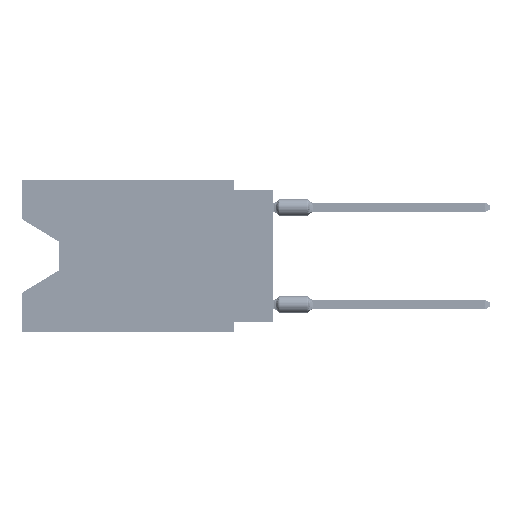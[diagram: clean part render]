
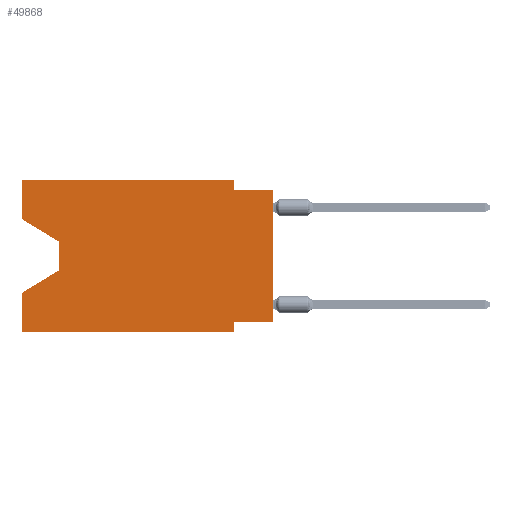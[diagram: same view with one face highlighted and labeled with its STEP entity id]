
A CAD part, left-side view. The second image highlights one B-rep face of the part: STEP entity #49868.
In plain terms, the highlighted planar face has unit normal (-1, 0, 0).
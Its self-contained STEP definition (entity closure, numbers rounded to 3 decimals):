
#768 = EDGE_CURVE ( 'NONE', #69960, #24962, #81163, .T. ) ;
#1006 = EDGE_CURVE ( 'NONE', #70549, #54076, #15546, .T. ) ;
#4411 = ORIENTED_EDGE ( 'NONE', *, *, #64118, .T. ) ;
#5309 = VECTOR ( 'NONE', #42907, 1000. ) ;
#5579 = CARTESIAN_POINT ( 'NONE',  ( 0., 2.54, -0.635 ) ) ;
#6968 = ORIENTED_EDGE ( 'NONE', *, *, #57797, .T. ) ;
#8284 = DIRECTION ( 'NONE',  ( 1., 0., 0. ) ) ;
#9071 = DIRECTION ( 'NONE',  ( 0., 0., -1. ) ) ;
#11226 = CARTESIAN_POINT ( 'NONE',  ( 0., 0., -0.635 ) ) ;
#12675 = VERTEX_POINT ( 'NONE', #26516 ) ;
#13913 = ORIENTED_EDGE ( 'NONE', *, *, #57870, .T. ) ;
#14040 = EDGE_CURVE ( 'NONE', #12675, #62823, #24757, .T. ) ;
#14303 = DIRECTION ( 'NONE',  ( 0., 1., 0. ) ) ;
#14999 = PLANE ( 'NONE',  #27653 ) ;
#15546 = LINE ( 'NONE', #59275, #26332 ) ;
#15620 = VECTOR ( 'NONE', #56709, 1000. ) ;
#15772 = VERTEX_POINT ( 'NONE', #11226 ) ;
#17292 = CARTESIAN_POINT ( 'NONE',  ( 0., 16.383, -9.906 ) ) ;
#17802 = CARTESIAN_POINT ( 'NONE',  ( 0., 13.97, -5.893 ) ) ;
#19247 = CARTESIAN_POINT ( 'NONE',  ( 0., 2.54, -9.906 ) ) ;
#19564 = LINE ( 'NONE', #26283, #22135 ) ;
#22135 = VECTOR ( 'NONE', #33429, 1000. ) ;
#23839 = DIRECTION ( 'NONE',  ( 0., 0., 1. ) ) ;
#24064 = VERTEX_POINT ( 'NONE', #17802 ) ;
#24757 = LINE ( 'NONE', #44124, #15620 ) ;
#24962 = VERTEX_POINT ( 'NONE', #19247 ) ;
#25573 = EDGE_CURVE ( 'NONE', #70549, #15772, #19564, .T. ) ;
#25638 = CARTESIAN_POINT ( 'NONE',  ( 0., 16.383, 0. ) ) ;
#25641 = LINE ( 'NONE', #70570, #53686 ) ;
#26283 = CARTESIAN_POINT ( 'NONE',  ( 0., 0., 0. ) ) ;
#26332 = VECTOR ( 'NONE', #14303, 1000. ) ;
#26516 = CARTESIAN_POINT ( 'NONE',  ( 0., 2.54, 0. ) ) ;
#27653 = AXIS2_PLACEMENT_3D ( 'NONE', #40669, #8284, #28854 ) ;
#28854 = DIRECTION ( 'NONE',  ( 0., 0., -1. ) ) ;
#29855 = LINE ( 'NONE', #55498, #5309 ) ;
#32883 = DIRECTION ( 'NONE',  ( 0., 0.855, -0.519 ) ) ;
#33429 = DIRECTION ( 'NONE',  ( 0., 0., 1. ) ) ;
#33769 = EDGE_CURVE ( 'NONE', #51291, #51063, #41152, .T. ) ;
#34732 = EDGE_CURVE ( 'NONE', #69960, #39085, #69340, .T. ) ;
#35984 = VERTEX_POINT ( 'NONE', #67940 ) ;
#38389 = ORIENTED_EDGE ( 'NONE', *, *, #25573, .T. ) ;
#39085 = VERTEX_POINT ( 'NONE', #78237 ) ;
#39200 = CARTESIAN_POINT ( 'NONE',  ( 0., 13.97, -5.893 ) ) ;
#40669 = CARTESIAN_POINT ( 'NONE',  ( 0., 16.383, 0. ) ) ;
#41152 = LINE ( 'NONE', #81413, #45690 ) ;
#42014 = VECTOR ( 'NONE', #80746, 1000. ) ;
#42800 = ORIENTED_EDGE ( 'NONE', *, *, #768, .T. ) ;
#42907 = DIRECTION ( 'NONE',  ( 0., -0.855, -0.519 ) ) ;
#43771 = VECTOR ( 'NONE', #61012, 1000. ) ;
#44076 = ORIENTED_EDGE ( 'NONE', *, *, #33769, .F. ) ;
#44124 = CARTESIAN_POINT ( 'NONE',  ( 0., 2.54, 0. ) ) ;
#44473 = ORIENTED_EDGE ( 'NONE', *, *, #80809, .F. ) ;
#44605 = EDGE_CURVE ( 'NONE', #62823, #15772, #48021, .T. ) ;
#45084 = ORIENTED_EDGE ( 'NONE', *, *, #34732, .F. ) ;
#45395 = DIRECTION ( 'NONE',  ( 0., 0., -1. ) ) ;
#45690 = VECTOR ( 'NONE', #23839, 1000. ) ;
#47388 = FACE_OUTER_BOUND ( 'NONE', #77397, .T. ) ;
#47866 = ORIENTED_EDGE ( 'NONE', *, *, #44605, .F. ) ;
#48021 = LINE ( 'NONE', #55122, #42014 ) ;
#48930 = CARTESIAN_POINT ( 'NONE',  ( 0., 16.383, 0. ) ) ;
#49868 = ADVANCED_FACE ( 'NONE', ( #47388 ), #14999, .F. ) ;
#51063 = VERTEX_POINT ( 'NONE', #65012 ) ;
#51291 = VERTEX_POINT ( 'NONE', #75471 ) ;
#53686 = VECTOR ( 'NONE', #45395, 1000. ) ;
#54076 = VERTEX_POINT ( 'NONE', #82957 ) ;
#55122 = CARTESIAN_POINT ( 'NONE',  ( 0., 0., -0.635 ) ) ;
#55498 = CARTESIAN_POINT ( 'NONE',  ( 0., 16.383, -2.546 ) ) ;
#56709 = DIRECTION ( 'NONE',  ( 0., 0., -1. ) ) ;
#57797 = EDGE_CURVE ( 'NONE', #51291, #35984, #29855, .T. ) ;
#57870 = EDGE_CURVE ( 'NONE', #35984, #24064, #25641, .T. ) ;
#58385 = DIRECTION ( 'NONE',  ( 0., 0., 1. ) ) ;
#59275 = CARTESIAN_POINT ( 'NONE',  ( 0., 0., -9.271 ) ) ;
#61012 = DIRECTION ( 'NONE',  ( 0., -1., 0. ) ) ;
#62537 = CARTESIAN_POINT ( 'NONE',  ( 0., 0., -9.271 ) ) ;
#62823 = VERTEX_POINT ( 'NONE', #5579 ) ;
#63287 = ORIENTED_EDGE ( 'NONE', *, *, #1006, .F. ) ;
#63966 = ORIENTED_EDGE ( 'NONE', *, *, #72462, .F. ) ;
#64118 = EDGE_CURVE ( 'NONE', #24064, #39085, #77415, .T. ) ;
#65012 = CARTESIAN_POINT ( 'NONE',  ( 0., 16.383, 0. ) ) ;
#66581 = DIRECTION ( 'NONE',  ( 0., -1., 0. ) ) ;
#66636 = CARTESIAN_POINT ( 'NONE',  ( 0., 2.54, -9.906 ) ) ;
#67940 = CARTESIAN_POINT ( 'NONE',  ( 0., 13.97, -4.013 ) ) ;
#68511 = CARTESIAN_POINT ( 'NONE',  ( 0., 16.383, -9.906 ) ) ;
#69340 = LINE ( 'NONE', #25638, #75282 ) ;
#69960 = VERTEX_POINT ( 'NONE', #68511 ) ;
#70343 = VECTOR ( 'NONE', #32883, 1000. ) ;
#70549 = VERTEX_POINT ( 'NONE', #62537 ) ;
#70570 = CARTESIAN_POINT ( 'NONE',  ( 0., 13.97, -4.013 ) ) ;
#72462 = EDGE_CURVE ( 'NONE', #51063, #12675, #80839, .T. ) ;
#72918 = VECTOR ( 'NONE', #9071, 1000. ) ;
#73367 = LINE ( 'NONE', #66636, #72918 ) ;
#75282 = VECTOR ( 'NONE', #58385, 1000. ) ;
#75471 = CARTESIAN_POINT ( 'NONE',  ( 0., 16.383, -2.546 ) ) ;
#77397 = EDGE_LOOP ( 'NONE', ( #6968, #13913, #4411, #45084, #42800, #44473, #63287, #38389, #47866, #78566, #63966, #44076 ) ) ;
#77415 = LINE ( 'NONE', #39200, #70343 ) ;
#77995 = VECTOR ( 'NONE', #66581, 1000. ) ;
#78237 = CARTESIAN_POINT ( 'NONE',  ( 0., 16.383, -7.36 ) ) ;
#78566 = ORIENTED_EDGE ( 'NONE', *, *, #14040, .F. ) ;
#80746 = DIRECTION ( 'NONE',  ( 0., -1., 0. ) ) ;
#80809 = EDGE_CURVE ( 'NONE', #54076, #24962, #73367, .T. ) ;
#80839 = LINE ( 'NONE', #48930, #77995 ) ;
#81163 = LINE ( 'NONE', #17292, #43771 ) ;
#81413 = CARTESIAN_POINT ( 'NONE',  ( 0., 16.383, 0. ) ) ;
#82957 = CARTESIAN_POINT ( 'NONE',  ( 0., 2.54, -9.271 ) ) ;
